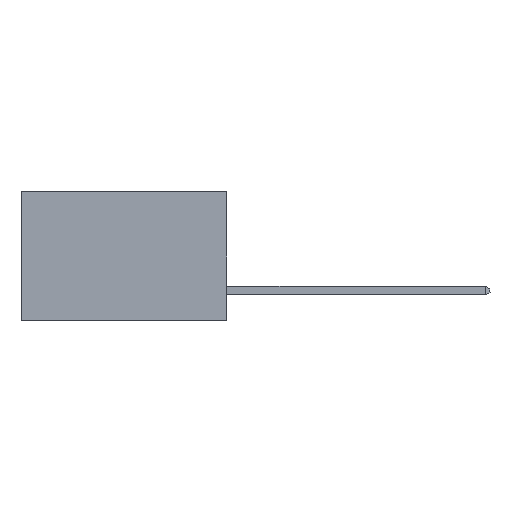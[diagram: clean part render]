
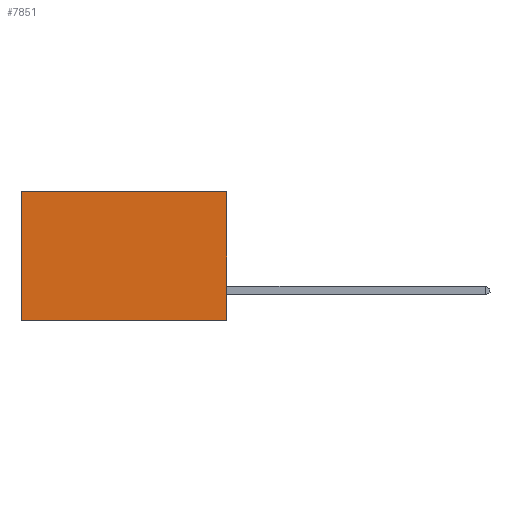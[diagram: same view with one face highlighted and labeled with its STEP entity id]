
A CAD part, left-side view. The second image highlights one B-rep face of the part: STEP entity #7851.
In plain terms, the highlighted planar face has unit normal (-1, 0, 0).
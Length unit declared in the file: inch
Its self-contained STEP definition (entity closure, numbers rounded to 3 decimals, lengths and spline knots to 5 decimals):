
#107 = DIRECTION ( 'NONE',  ( 0., 0., -1. ) ) ;
#852 = VERTEX_POINT ( 'NONE', #5953 ) ;
#896 = VERTEX_POINT ( 'NONE', #7047 ) ;
#1430 = EDGE_LOOP ( 'NONE', ( #4467, #12363, #9586, #16857 ) ) ;
#1773 = PLANE ( 'NONE',  #2122 ) ;
#2122 = AXIS2_PLACEMENT_3D ( 'NONE', #14551, #6177, #15932 ) ;
#3182 = EDGE_CURVE ( 'NONE', #4558, #852, #8185, .T. ) ;
#3254 = CARTESIAN_POINT ( 'NONE',  ( 0.277, 0., 0. ) ) ;
#3884 = VECTOR ( 'NONE', #107, 39.37008 ) ;
#4467 = ORIENTED_EDGE ( 'NONE', *, *, #3182, .T. ) ;
#4558 = VERTEX_POINT ( 'NONE', #16035 ) ;
#4572 = LINE ( 'NONE', #15181, #15353 ) ;
#5953 = CARTESIAN_POINT ( 'NONE',  ( 0.277, 0.59, -0.37 ) ) ;
#6177 = DIRECTION ( 'NONE',  ( 1., 0., 0. ) ) ;
#7047 = CARTESIAN_POINT ( 'NONE',  ( 0.277, 0., 0. ) ) ;
#7851 = ADVANCED_FACE ( 'NONE', ( #15614 ), #1773, .F. ) ;
#8185 = LINE ( 'NONE', #10165, #3884 ) ;
#8255 = LINE ( 'NONE', #3254, #8684 ) ;
#8636 = DIRECTION ( 'NONE',  ( 0., 0., -1. ) ) ;
#8684 = VECTOR ( 'NONE', #10383, 39.37008 ) ;
#8822 = VERTEX_POINT ( 'NONE', #16440 ) ;
#8849 = EDGE_CURVE ( 'NONE', #8822, #852, #4572, .T. ) ;
#9586 = ORIENTED_EDGE ( 'NONE', *, *, #15376, .F. ) ;
#10165 = CARTESIAN_POINT ( 'NONE',  ( 0.277, 0.59, -0.37 ) ) ;
#10383 = DIRECTION ( 'NONE',  ( 0., 1., 0. ) ) ;
#11063 = DIRECTION ( 'NONE',  ( 0., 1., 0. ) ) ;
#11698 = EDGE_CURVE ( 'NONE', #896, #4558, #8255, .T. ) ;
#12363 = ORIENTED_EDGE ( 'NONE', *, *, #8849, .F. ) ;
#13368 = VECTOR ( 'NONE', #8636, 39.37008 ) ;
#14198 = CARTESIAN_POINT ( 'NONE',  ( 0.277, 0., -0.37 ) ) ;
#14551 = CARTESIAN_POINT ( 'NONE',  ( 0.277, 0., -0.37 ) ) ;
#15181 = CARTESIAN_POINT ( 'NONE',  ( 0.277, 0., -0.37 ) ) ;
#15353 = VECTOR ( 'NONE', #11063, 39.37008 ) ;
#15376 = EDGE_CURVE ( 'NONE', #896, #8822, #17048, .T. ) ;
#15614 = FACE_OUTER_BOUND ( 'NONE', #1430, .T. ) ;
#15932 = DIRECTION ( 'NONE',  ( 0., 0., -1. ) ) ;
#16035 = CARTESIAN_POINT ( 'NONE',  ( 0.277, 0.59, 0. ) ) ;
#16440 = CARTESIAN_POINT ( 'NONE',  ( 0.277, 0., -0.37 ) ) ;
#16857 = ORIENTED_EDGE ( 'NONE', *, *, #11698, .T. ) ;
#17048 = LINE ( 'NONE', #14198, #13368 ) ;
